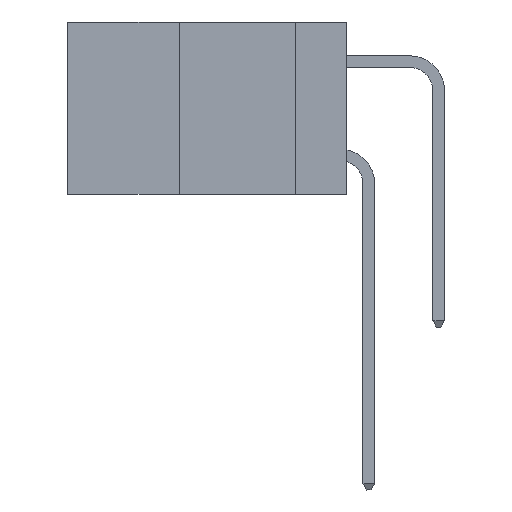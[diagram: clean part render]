
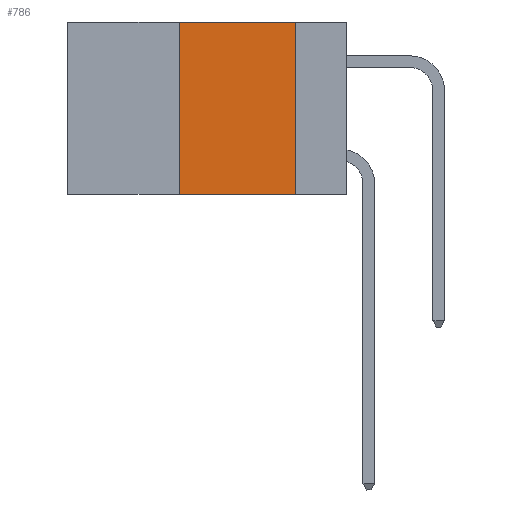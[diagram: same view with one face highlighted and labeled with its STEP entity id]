
A CAD part, left-side view. The second image highlights one B-rep face of the part: STEP entity #786.
In plain terms, the highlighted planar face has unit normal (-1, 0, 0).
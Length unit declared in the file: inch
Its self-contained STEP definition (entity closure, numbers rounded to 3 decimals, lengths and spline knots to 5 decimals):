
#786 = ADVANCED_FACE ( 'NONE', ( #6052 ), #6050, .F. ) ;
#1554 = VERTEX_POINT ( 'NONE', #3630 ) ;
#1678 = CARTESIAN_POINT ( 'NONE',  ( 0., 0.6, -0.37 ) ) ;
#1715 = DIRECTION ( 'NONE',  ( 0., -1., 0. ) ) ;
#1844 = VERTEX_POINT ( 'NONE', #11076 ) ;
#2142 = VERTEX_POINT ( 'NONE', #2710 ) ;
#2205 = VERTEX_POINT ( 'NONE', #6696 ) ;
#2351 = CARTESIAN_POINT ( 'NONE',  ( 0., 0.36, 0. ) ) ;
#2566 = DIRECTION ( 'NONE',  ( 0., -1., 0. ) ) ;
#2710 = CARTESIAN_POINT ( 'NONE',  ( 0., 0.11, 0. ) ) ;
#3368 = EDGE_CURVE ( 'NONE', #1554, #1844, #10519, .T. ) ;
#3630 = CARTESIAN_POINT ( 'NONE',  ( 0., 0.36, -0.37 ) ) ;
#4026 = DIRECTION ( 'NONE',  ( 0., 0., -1. ) ) ;
#4122 = VECTOR ( 'NONE', #9193, 39.37008 ) ;
#4493 = ORIENTED_EDGE ( 'NONE', *, *, #3368, .F. ) ;
#4792 = DIRECTION ( 'NONE',  ( 1., 0., 0. ) ) ;
#4921 = EDGE_LOOP ( 'NONE', ( #6818, #8059, #4493, #9935 ) ) ;
#5127 = AXIS2_PLACEMENT_3D ( 'NONE', #5698, #4792, #4026 ) ;
#5593 = EDGE_CURVE ( 'NONE', #2142, #2205, #6752, .T. ) ;
#5698 = CARTESIAN_POINT ( 'NONE',  ( 0., 0.6, 0. ) ) ;
#6050 = PLANE ( 'NONE',  #5127 ) ;
#6052 = FACE_OUTER_BOUND ( 'NONE', #4921, .T. ) ;
#6125 = VECTOR ( 'NONE', #8088, 39.37008 ) ;
#6696 = CARTESIAN_POINT ( 'NONE',  ( 0., 0.11, -0.37 ) ) ;
#6752 = LINE ( 'NONE', #10007, #4122 ) ;
#6818 = ORIENTED_EDGE ( 'NONE', *, *, #5593, .F. ) ;
#7458 = EDGE_CURVE ( 'NONE', #1844, #2142, #9869, .T. ) ;
#7715 = VECTOR ( 'NONE', #1715, 39.37008 ) ;
#8044 = LINE ( 'NONE', #1678, #9676 ) ;
#8059 = ORIENTED_EDGE ( 'NONE', *, *, #7458, .F. ) ;
#8088 = DIRECTION ( 'NONE',  ( 0., 0., 1. ) ) ;
#9193 = DIRECTION ( 'NONE',  ( 0., 0., -1. ) ) ;
#9550 = CARTESIAN_POINT ( 'NONE',  ( 0., 0.6, 0. ) ) ;
#9676 = VECTOR ( 'NONE', #2566, 39.37008 ) ;
#9869 = LINE ( 'NONE', #9550, #7715 ) ;
#9935 = ORIENTED_EDGE ( 'NONE', *, *, #10444, .T. ) ;
#10007 = CARTESIAN_POINT ( 'NONE',  ( 0., 0.11, 0. ) ) ;
#10444 = EDGE_CURVE ( 'NONE', #1554, #2205, #8044, .T. ) ;
#10519 = LINE ( 'NONE', #2351, #6125 ) ;
#11076 = CARTESIAN_POINT ( 'NONE',  ( 0., 0.36, 0. ) ) ;
